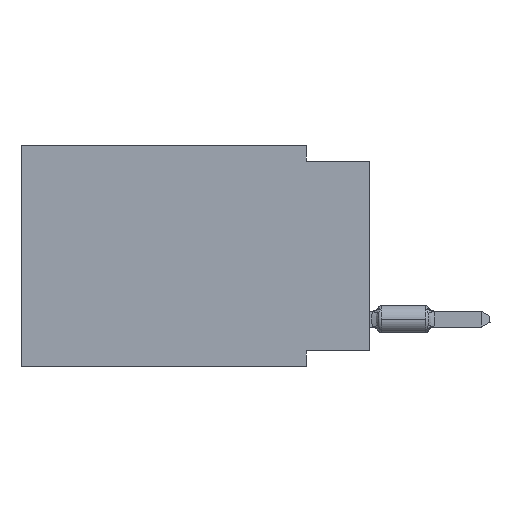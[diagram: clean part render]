
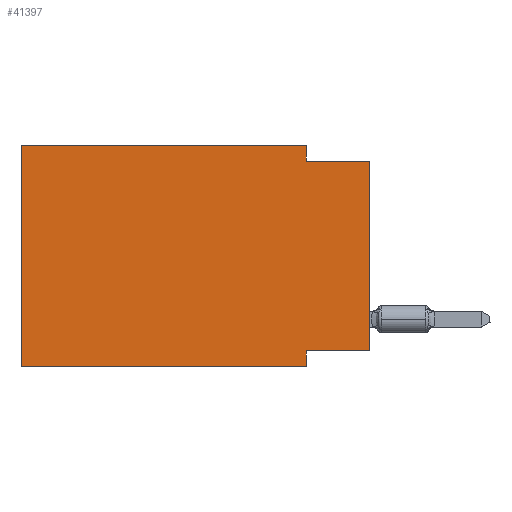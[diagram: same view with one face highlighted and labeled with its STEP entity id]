
A CAD part, left-side view. The second image highlights one B-rep face of the part: STEP entity #41397.
In plain terms, the highlighted planar face has unit normal (-1, 0, 0).
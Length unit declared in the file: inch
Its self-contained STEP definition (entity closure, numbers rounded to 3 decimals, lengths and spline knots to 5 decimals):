
#726 = LINE ( 'NONE', #21389, #51995 ) ;
#986 = AXIS2_PLACEMENT_3D ( 'NONE', #42346, #37763, #43005 ) ;
#1162 = EDGE_CURVE ( 'NONE', #19968, #39344, #1194, .T. ) ;
#1194 = LINE ( 'NONE', #56273, #23604 ) ;
#1792 = LINE ( 'NONE', #42413, #12221 ) ;
#2712 = CARTESIAN_POINT ( 'NONE',  ( 0., 0.1, -0.35 ) ) ;
#2825 = DIRECTION ( 'NONE',  ( 0., -1., 0. ) ) ;
#3413 = DIRECTION ( 'NONE',  ( 0., -1., 0. ) ) ;
#5511 = CARTESIAN_POINT ( 'NONE',  ( 0., 0., -0.025 ) ) ;
#6498 = CARTESIAN_POINT ( 'NONE',  ( 0., 0.1, -0.325 ) ) ;
#7209 = VERTEX_POINT ( 'NONE', #9523 ) ;
#7535 = VERTEX_POINT ( 'NONE', #13062 ) ;
#8052 = EDGE_CURVE ( 'NONE', #61922, #7209, #34929, .T. ) ;
#8798 = CARTESIAN_POINT ( 'NONE',  ( 0., 0.55, 0. ) ) ;
#9523 = CARTESIAN_POINT ( 'NONE',  ( 0., 0.55, 0. ) ) ;
#12221 = VECTOR ( 'NONE', #12597, 39.37008 ) ;
#12597 = DIRECTION ( 'NONE',  ( 0., 0., -1. ) ) ;
#13062 = CARTESIAN_POINT ( 'NONE',  ( 0., 0.1, 0. ) ) ;
#19968 = VERTEX_POINT ( 'NONE', #35839 ) ;
#20962 = ORIENTED_EDGE ( 'NONE', *, *, #63976, .F. ) ;
#21389 = CARTESIAN_POINT ( 'NONE',  ( 0., 0.1, 0. ) ) ;
#21943 = ORIENTED_EDGE ( 'NONE', *, *, #55350, .F. ) ;
#22851 = LINE ( 'NONE', #62445, #48464 ) ;
#23604 = VECTOR ( 'NONE', #41511, 39.37008 ) ;
#24261 = CARTESIAN_POINT ( 'NONE',  ( 0., 0., 0. ) ) ;
#25116 = DIRECTION ( 'NONE',  ( 0., 0., 1. ) ) ;
#28355 = LINE ( 'NONE', #48309, #34157 ) ;
#28755 = ORIENTED_EDGE ( 'NONE', *, *, #51698, .T. ) ;
#30359 = CARTESIAN_POINT ( 'NONE',  ( 0., 0.55, 0. ) ) ;
#31303 = ORIENTED_EDGE ( 'NONE', *, *, #8052, .F. ) ;
#32047 = VECTOR ( 'NONE', #39580, 39.37008 ) ;
#34084 = LINE ( 'NONE', #24261, #63716 ) ;
#34157 = VECTOR ( 'NONE', #3413, 39.37008 ) ;
#34929 = LINE ( 'NONE', #30359, #60971 ) ;
#35839 = CARTESIAN_POINT ( 'NONE',  ( 0., 0., -0.325 ) ) ;
#36722 = EDGE_CURVE ( 'NONE', #7535, #59887, #726, .T. ) ;
#37763 = DIRECTION ( 'NONE',  ( 1., 0., 0. ) ) ;
#38559 = EDGE_CURVE ( 'NONE', #39344, #57868, #1792, .T. ) ;
#39344 = VERTEX_POINT ( 'NONE', #6498 ) ;
#39580 = DIRECTION ( 'NONE',  ( 0., -1., 0. ) ) ;
#40755 = EDGE_CURVE ( 'NONE', #19968, #62019, #34084, .T. ) ;
#41352 = DIRECTION ( 'NONE',  ( 0., 0., -1. ) ) ;
#41397 = ADVANCED_FACE ( 'NONE', ( #53172 ), #57104, .F. ) ;
#41511 = DIRECTION ( 'NONE',  ( 0., 1., 0. ) ) ;
#42346 = CARTESIAN_POINT ( 'NONE',  ( 0., 0.55, 0. ) ) ;
#42413 = CARTESIAN_POINT ( 'NONE',  ( 0., 0.1, -0.35 ) ) ;
#42705 = ORIENTED_EDGE ( 'NONE', *, *, #1162, .F. ) ;
#43005 = DIRECTION ( 'NONE',  ( 0., 0., -1. ) ) ;
#46696 = ORIENTED_EDGE ( 'NONE', *, *, #36722, .F. ) ;
#48309 = CARTESIAN_POINT ( 'NONE',  ( 0., 0., -0.025 ) ) ;
#48464 = VECTOR ( 'NONE', #2825, 39.37008 ) ;
#48699 = EDGE_LOOP ( 'NONE', ( #53029, #20962, #46696, #21943, #31303, #28755, #57790, #42705 ) ) ;
#48793 = CARTESIAN_POINT ( 'NONE',  ( 0., 0.55, -0.35 ) ) ;
#51698 = EDGE_CURVE ( 'NONE', #61922, #57868, #22851, .T. ) ;
#51995 = VECTOR ( 'NONE', #41352, 39.37008 ) ;
#53029 = ORIENTED_EDGE ( 'NONE', *, *, #40755, .T. ) ;
#53172 = FACE_OUTER_BOUND ( 'NONE', #48699, .T. ) ;
#55350 = EDGE_CURVE ( 'NONE', #7209, #7535, #58918, .T. ) ;
#56273 = CARTESIAN_POINT ( 'NONE',  ( 0., 0., -0.325 ) ) ;
#57104 = PLANE ( 'NONE',  #986 ) ;
#57790 = ORIENTED_EDGE ( 'NONE', *, *, #38559, .F. ) ;
#57868 = VERTEX_POINT ( 'NONE', #2712 ) ;
#58918 = LINE ( 'NONE', #8798, #32047 ) ;
#59887 = VERTEX_POINT ( 'NONE', #61561 ) ;
#60971 = VECTOR ( 'NONE', #25116, 39.37008 ) ;
#61561 = CARTESIAN_POINT ( 'NONE',  ( 0., 0.1, -0.025 ) ) ;
#61922 = VERTEX_POINT ( 'NONE', #48793 ) ;
#62019 = VERTEX_POINT ( 'NONE', #5511 ) ;
#62445 = CARTESIAN_POINT ( 'NONE',  ( 0., 0.55, -0.35 ) ) ;
#63716 = VECTOR ( 'NONE', #64174, 39.37008 ) ;
#63976 = EDGE_CURVE ( 'NONE', #59887, #62019, #28355, .T. ) ;
#64174 = DIRECTION ( 'NONE',  ( 0., 0., 1. ) ) ;
